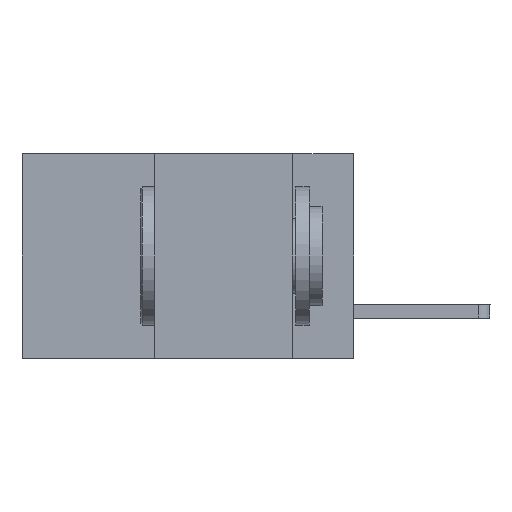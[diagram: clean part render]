
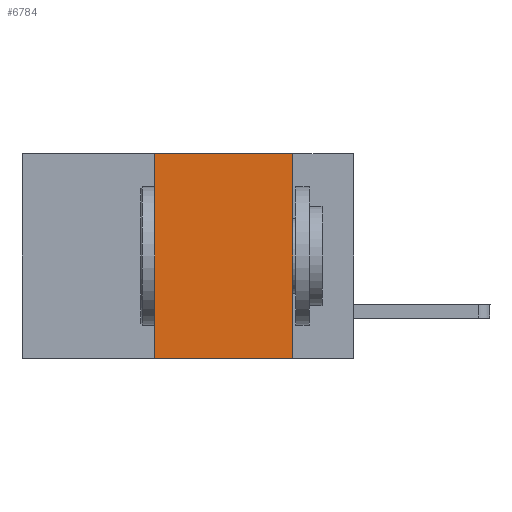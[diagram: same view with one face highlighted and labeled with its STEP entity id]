
A CAD part, left-side view. The second image highlights one B-rep face of the part: STEP entity #6784.
In plain terms, the highlighted planar face has unit normal (-1, 0, 0).
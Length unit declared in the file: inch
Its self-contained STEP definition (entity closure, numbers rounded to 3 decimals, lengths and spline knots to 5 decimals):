
#164 = EDGE_CURVE ( 'NONE', #5784, #2249, #1569, .T. ) ;
#320 = VERTEX_POINT ( 'NONE', #7949 ) ;
#671 = EDGE_LOOP ( 'NONE', ( #7074, #2739, #7094, #2425 ) ) ;
#1031 = CARTESIAN_POINT ( 'NONE',  ( 0., 0.6, -0.37 ) ) ;
#1569 = LINE ( 'NONE', #8644, #2070 ) ;
#1572 = DIRECTION ( 'NONE',  ( 0., 0., -1. ) ) ;
#2070 = VECTOR ( 'NONE', #1572, 39.37008 ) ;
#2249 = VERTEX_POINT ( 'NONE', #4710 ) ;
#2425 = ORIENTED_EDGE ( 'NONE', *, *, #6608, .T. ) ;
#2739 = ORIENTED_EDGE ( 'NONE', *, *, #4193, .F. ) ;
#2790 = CARTESIAN_POINT ( 'NONE',  ( 0., 0.6, 0. ) ) ;
#2883 = CARTESIAN_POINT ( 'NONE',  ( 0., 0.6, 0. ) ) ;
#2908 = LINE ( 'NONE', #1031, #9028 ) ;
#4193 = EDGE_CURVE ( 'NONE', #320, #5784, #5193, .T. ) ;
#4423 = VERTEX_POINT ( 'NONE', #6096 ) ;
#4710 = CARTESIAN_POINT ( 'NONE',  ( 0., 0.11, -0.37 ) ) ;
#4920 = DIRECTION ( 'NONE',  ( 0., -1., 0. ) ) ;
#5142 = VECTOR ( 'NONE', #5549, 39.37008 ) ;
#5193 = LINE ( 'NONE', #2790, #6521 ) ;
#5549 = DIRECTION ( 'NONE',  ( 0., 0., 1. ) ) ;
#5784 = VERTEX_POINT ( 'NONE', #6239 ) ;
#6050 = PLANE ( 'NONE',  #9696 ) ;
#6093 = EDGE_CURVE ( 'NONE', #4423, #320, #9484, .T. ) ;
#6096 = CARTESIAN_POINT ( 'NONE',  ( 0., 0.36, -0.37 ) ) ;
#6239 = CARTESIAN_POINT ( 'NONE',  ( 0., 0.11, 0. ) ) ;
#6521 = VECTOR ( 'NONE', #8277, 39.37008 ) ;
#6608 = EDGE_CURVE ( 'NONE', #4423, #2249, #2908, .T. ) ;
#6784 = ADVANCED_FACE ( 'NONE', ( #9969 ), #6050, .F. ) ;
#7074 = ORIENTED_EDGE ( 'NONE', *, *, #164, .F. ) ;
#7094 = ORIENTED_EDGE ( 'NONE', *, *, #6093, .F. ) ;
#7943 = CARTESIAN_POINT ( 'NONE',  ( 0., 0.36, 0. ) ) ;
#7949 = CARTESIAN_POINT ( 'NONE',  ( 0., 0.36, 0. ) ) ;
#8277 = DIRECTION ( 'NONE',  ( 0., -1., 0. ) ) ;
#8345 = DIRECTION ( 'NONE',  ( 1., 0., 0. ) ) ;
#8644 = CARTESIAN_POINT ( 'NONE',  ( 0., 0.11, 0. ) ) ;
#9028 = VECTOR ( 'NONE', #4920, 39.37008 ) ;
#9136 = DIRECTION ( 'NONE',  ( 0., 0., -1. ) ) ;
#9484 = LINE ( 'NONE', #7943, #5142 ) ;
#9696 = AXIS2_PLACEMENT_3D ( 'NONE', #2883, #8345, #9136 ) ;
#9969 = FACE_OUTER_BOUND ( 'NONE', #671, .T. ) ;
